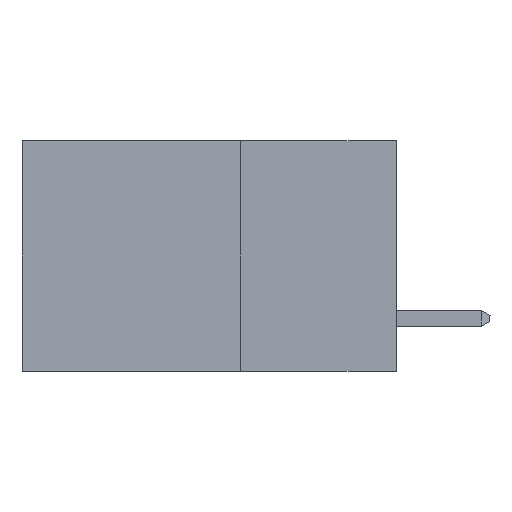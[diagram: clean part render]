
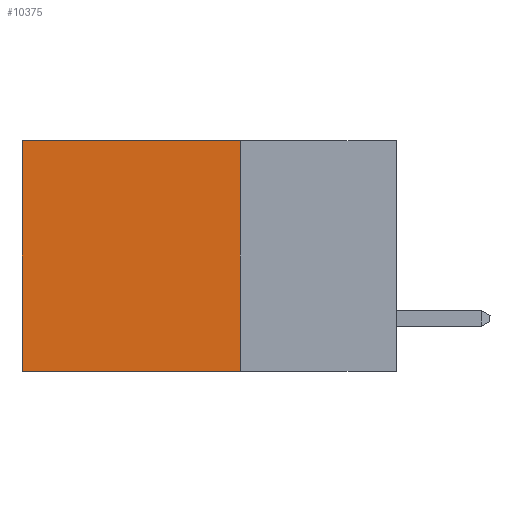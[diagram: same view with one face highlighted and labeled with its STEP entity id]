
A CAD part, left-side view. The second image highlights one B-rep face of the part: STEP entity #10375.
In plain terms, the highlighted planar face has unit normal (-1, 0, 0).
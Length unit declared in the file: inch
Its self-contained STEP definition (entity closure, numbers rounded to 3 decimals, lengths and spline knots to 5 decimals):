
#296 = EDGE_CURVE ( 'NONE', #1352, #14805, #5709, .T. ) ;
#443 = EDGE_LOOP ( 'NONE', ( #19146, #4965, #4832, #5633 ) ) ;
#570 = CARTESIAN_POINT ( 'NONE',  ( 0.298, 0.6, -0.37 ) ) ;
#959 = VERTEX_POINT ( 'NONE', #19143 ) ;
#1303 = VECTOR ( 'NONE', #12052, 39.37008 ) ;
#1352 = VERTEX_POINT ( 'NONE', #14483 ) ;
#2782 = LINE ( 'NONE', #5685, #18387 ) ;
#4832 = ORIENTED_EDGE ( 'NONE', *, *, #6018, .F. ) ;
#4965 = ORIENTED_EDGE ( 'NONE', *, *, #296, .F. ) ;
#5085 = DIRECTION ( 'NONE',  ( 0., 1., 0. ) ) ;
#5254 = VERTEX_POINT ( 'NONE', #17154 ) ;
#5633 = ORIENTED_EDGE ( 'NONE', *, *, #9543, .T. ) ;
#5682 = CARTESIAN_POINT ( 'NONE',  ( 0.298, 0.25, 0. ) ) ;
#5685 = CARTESIAN_POINT ( 'NONE',  ( 0.298, 0.6, 0. ) ) ;
#5709 = LINE ( 'NONE', #14143, #9281 ) ;
#5871 = DIRECTION ( 'NONE',  ( 0., 0., -1. ) ) ;
#6018 = EDGE_CURVE ( 'NONE', #959, #1352, #18247, .T. ) ;
#6175 = VECTOR ( 'NONE', #13158, 39.37008 ) ;
#7160 = PLANE ( 'NONE',  #12604 ) ;
#9049 = EDGE_CURVE ( 'NONE', #5254, #14805, #2782, .T. ) ;
#9281 = VECTOR ( 'NONE', #5085, 39.37008 ) ;
#9543 = EDGE_CURVE ( 'NONE', #959, #5254, #15781, .T. ) ;
#10375 = ADVANCED_FACE ( 'NONE', ( #12151 ), #7160, .F. ) ;
#12052 = DIRECTION ( 'NONE',  ( 0., 1., 0. ) ) ;
#12151 = FACE_OUTER_BOUND ( 'NONE', #443, .T. ) ;
#12604 = AXIS2_PLACEMENT_3D ( 'NONE', #5682, #17736, #5871 ) ;
#13158 = DIRECTION ( 'NONE',  ( 0., 0., -1. ) ) ;
#14143 = CARTESIAN_POINT ( 'NONE',  ( 0.298, 0.25, -0.37 ) ) ;
#14483 = CARTESIAN_POINT ( 'NONE',  ( 0.298, 0.25, -0.37 ) ) ;
#14805 = VERTEX_POINT ( 'NONE', #570 ) ;
#14921 = CARTESIAN_POINT ( 'NONE',  ( 0.298, 0.25, 0. ) ) ;
#15781 = LINE ( 'NONE', #14921, #1303 ) ;
#16152 = CARTESIAN_POINT ( 'NONE',  ( 0.298, 0.25, 0. ) ) ;
#17154 = CARTESIAN_POINT ( 'NONE',  ( 0.298, 0.6, 0. ) ) ;
#17736 = DIRECTION ( 'NONE',  ( 1., 0., 0. ) ) ;
#17806 = DIRECTION ( 'NONE',  ( 0., 0., -1. ) ) ;
#18247 = LINE ( 'NONE', #16152, #6175 ) ;
#18387 = VECTOR ( 'NONE', #17806, 39.37008 ) ;
#19143 = CARTESIAN_POINT ( 'NONE',  ( 0.298, 0.25, 0. ) ) ;
#19146 = ORIENTED_EDGE ( 'NONE', *, *, #9049, .T. ) ;
